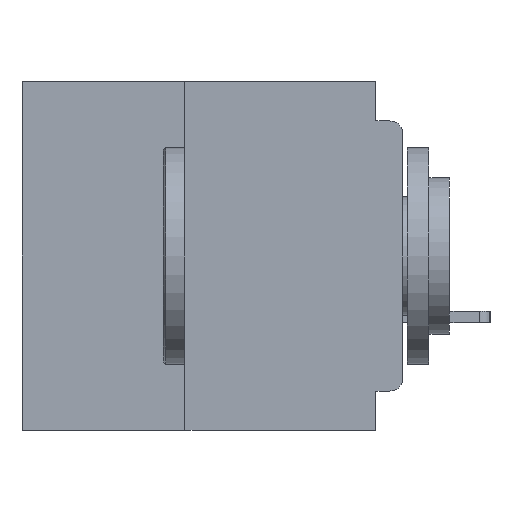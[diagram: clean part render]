
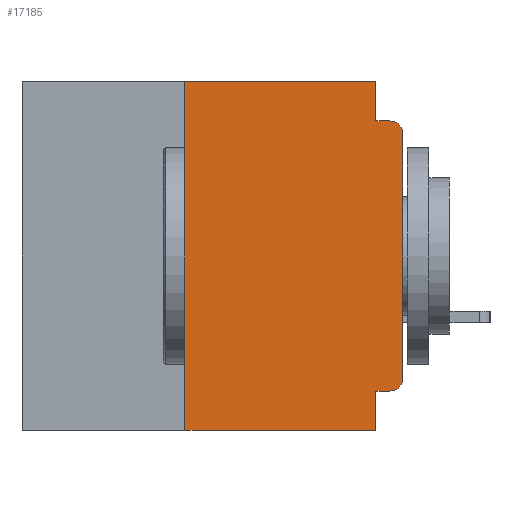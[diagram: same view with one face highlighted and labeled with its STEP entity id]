
A CAD part, left-side view. The second image highlights one B-rep face of the part: STEP entity #17185.
In plain terms, the highlighted planar face has unit normal (-1, 0, 0).
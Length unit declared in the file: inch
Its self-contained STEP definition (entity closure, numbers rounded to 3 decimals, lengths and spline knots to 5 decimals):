
#97 = VERTEX_POINT ( 'NONE', #34291 ) ;
#770 = CARTESIAN_POINT ( 'NONE',  ( 0., 0.015, -0.34 ) ) ;
#1156 = ORIENTED_EDGE ( 'NONE', *, *, #6520, .F. ) ;
#1467 = LINE ( 'NONE', #35261, #7687 ) ;
#1502 = ORIENTED_EDGE ( 'NONE', *, *, #7130, .T. ) ;
#1866 = AXIS2_PLACEMENT_3D ( 'NONE', #22015, #3978, #13113 ) ;
#2853 = EDGE_CURVE ( 'NONE', #97, #10696, #4100, .T. ) ;
#2902 = VERTEX_POINT ( 'NONE', #10221 ) ;
#3189 = EDGE_CURVE ( 'NONE', #26302, #16019, #22923, .T. ) ;
#3239 = DIRECTION ( 'NONE',  ( 0., 0., 1. ) ) ;
#3835 = DIRECTION ( 'NONE',  ( 0., 0., -1. ) ) ;
#3863 = FACE_OUTER_BOUND ( 'NONE', #31201, .T. ) ;
#3978 = DIRECTION ( 'NONE',  ( 1., 0., 0. ) ) ;
#4100 = LINE ( 'NONE', #12395, #35234 ) ;
#4398 = VECTOR ( 'NONE', #3239, 39.37008 ) ;
#4433 = EDGE_CURVE ( 'NONE', #27587, #8774, #24711, .T. ) ;
#5044 = CARTESIAN_POINT ( 'NONE',  ( 0., 0.437, -0.4 ) ) ;
#5456 = CARTESIAN_POINT ( 'NONE',  ( 0., 0.015, -0.355 ) ) ;
#5892 = ORIENTED_EDGE ( 'NONE', *, *, #13661, .F. ) ;
#6520 = EDGE_CURVE ( 'NONE', #16811, #27587, #1467, .T. ) ;
#6808 = VECTOR ( 'NONE', #28399, 39.37008 ) ;
#6957 = ORIENTED_EDGE ( 'NONE', *, *, #30937, .T. ) ;
#7075 = CARTESIAN_POINT ( 'NONE',  ( 0., 0.031, -0.045 ) ) ;
#7130 = EDGE_CURVE ( 'NONE', #2902, #10696, #23568, .T. ) ;
#7289 = CARTESIAN_POINT ( 'NONE',  ( 0., 0., -0.34 ) ) ;
#7687 = VECTOR ( 'NONE', #11173, 39.37008 ) ;
#7769 = LINE ( 'NONE', #25378, #6808 ) ;
#8746 = VECTOR ( 'NONE', #37339, 39.37008 ) ;
#8774 = VERTEX_POINT ( 'NONE', #7075 ) ;
#9011 = VECTOR ( 'NONE', #19270, 39.37008 ) ;
#9027 = ORIENTED_EDGE ( 'NONE', *, *, #15493, .T. ) ;
#9936 = LINE ( 'NONE', #37333, #9011 ) ;
#10221 = CARTESIAN_POINT ( 'NONE',  ( 0., 0.25, -0.4 ) ) ;
#10696 = VERTEX_POINT ( 'NONE', #11960 ) ;
#11173 = DIRECTION ( 'NONE',  ( 0., -1., 0. ) ) ;
#11220 = AXIS2_PLACEMENT_3D ( 'NONE', #16538, #37572, #19512 ) ;
#11960 = CARTESIAN_POINT ( 'NONE',  ( 0., 0.031, -0.4 ) ) ;
#12345 = DIRECTION ( 'NONE',  ( 0., 0., -1. ) ) ;
#12383 = CARTESIAN_POINT ( 'NONE',  ( 0., 0.25, -0.4 ) ) ;
#12395 = CARTESIAN_POINT ( 'NONE',  ( 0., 0.031, -0.4 ) ) ;
#12868 = ORIENTED_EDGE ( 'NONE', *, *, #4433, .F. ) ;
#13113 = DIRECTION ( 'NONE',  ( 0., 0., -1. ) ) ;
#13661 = EDGE_CURVE ( 'NONE', #8774, #17215, #9936, .T. ) ;
#14576 = CARTESIAN_POINT ( 'NONE',  ( 0., 0., -0.06 ) ) ;
#15493 = EDGE_CURVE ( 'NONE', #30280, #17215, #37988, .T. ) ;
#16019 = VERTEX_POINT ( 'NONE', #7289 ) ;
#16538 = CARTESIAN_POINT ( 'NONE',  ( 0., 0.015, -0.06 ) ) ;
#16811 = VERTEX_POINT ( 'NONE', #17218 ) ;
#17185 = ADVANCED_FACE ( 'NONE', ( #3863 ), #31151, .F. ) ;
#17215 = VERTEX_POINT ( 'NONE', #37310 ) ;
#17218 = CARTESIAN_POINT ( 'NONE',  ( 0., 0.25, 0. ) ) ;
#19059 = VECTOR ( 'NONE', #26779, 39.37008 ) ;
#19270 = DIRECTION ( 'NONE',  ( 0., -1., 0. ) ) ;
#19512 = DIRECTION ( 'NONE',  ( 0., 0., -1. ) ) ;
#19867 = EDGE_CURVE ( 'NONE', #2902, #16811, #27507, .T. ) ;
#20256 = ORIENTED_EDGE ( 'NONE', *, *, #3189, .T. ) ;
#21863 = DIRECTION ( 'NONE',  ( -1., 0., 0. ) ) ;
#22015 = CARTESIAN_POINT ( 'NONE',  ( 0., 0.437, 0. ) ) ;
#22352 = ORIENTED_EDGE ( 'NONE', *, *, #26073, .F. ) ;
#22923 = CIRCLE ( 'NONE', #24753, 0.015 ) ;
#23568 = LINE ( 'NONE', #5044, #29714 ) ;
#24711 = LINE ( 'NONE', #25385, #8746 ) ;
#24753 = AXIS2_PLACEMENT_3D ( 'NONE', #770, #21863, #3835 ) ;
#25378 = CARTESIAN_POINT ( 'NONE',  ( 0., 0., -0.355 ) ) ;
#25385 = CARTESIAN_POINT ( 'NONE',  ( 0., 0.031, 0. ) ) ;
#26073 = EDGE_CURVE ( 'NONE', #26302, #97, #7769, .T. ) ;
#26302 = VERTEX_POINT ( 'NONE', #5456 ) ;
#26779 = DIRECTION ( 'NONE',  ( 0., 0., 1. ) ) ;
#27108 = LINE ( 'NONE', #29660, #19059 ) ;
#27507 = LINE ( 'NONE', #12383, #4398 ) ;
#27587 = VERTEX_POINT ( 'NONE', #33022 ) ;
#28006 = ORIENTED_EDGE ( 'NONE', *, *, #2853, .F. ) ;
#28399 = DIRECTION ( 'NONE',  ( 0., 1., 0. ) ) ;
#29156 = DIRECTION ( 'NONE',  ( 0., -1., 0. ) ) ;
#29660 = CARTESIAN_POINT ( 'NONE',  ( 0., 0., 0. ) ) ;
#29714 = VECTOR ( 'NONE', #29156, 39.37008 ) ;
#30280 = VERTEX_POINT ( 'NONE', #14576 ) ;
#30937 = EDGE_CURVE ( 'NONE', #16019, #30280, #27108, .T. ) ;
#31151 = PLANE ( 'NONE',  #1866 ) ;
#31201 = EDGE_LOOP ( 'NONE', ( #6957, #9027, #5892, #12868, #1156, #37100, #1502, #28006, #22352, #20256 ) ) ;
#33022 = CARTESIAN_POINT ( 'NONE',  ( 0., 0.031, 0. ) ) ;
#34291 = CARTESIAN_POINT ( 'NONE',  ( 0., 0.031, -0.355 ) ) ;
#35234 = VECTOR ( 'NONE', #12345, 39.37008 ) ;
#35261 = CARTESIAN_POINT ( 'NONE',  ( 0., 0.437, 0. ) ) ;
#37100 = ORIENTED_EDGE ( 'NONE', *, *, #19867, .F. ) ;
#37310 = CARTESIAN_POINT ( 'NONE',  ( 0., 0.015, -0.045 ) ) ;
#37333 = CARTESIAN_POINT ( 'NONE',  ( 0., 0., -0.045 ) ) ;
#37339 = DIRECTION ( 'NONE',  ( 0., 0., -1. ) ) ;
#37572 = DIRECTION ( 'NONE',  ( -1., 0., 0. ) ) ;
#37988 = CIRCLE ( 'NONE', #11220, 0.015 ) ;
